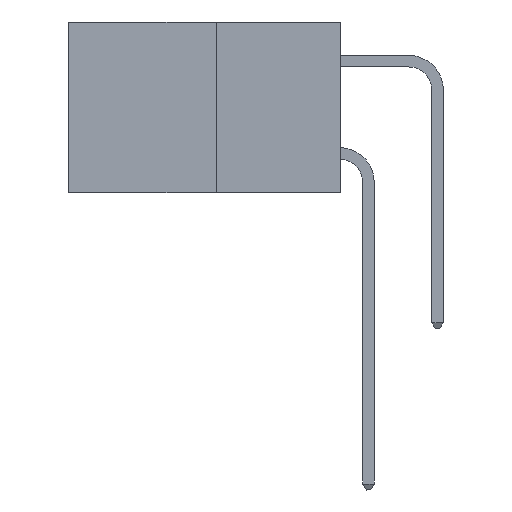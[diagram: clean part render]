
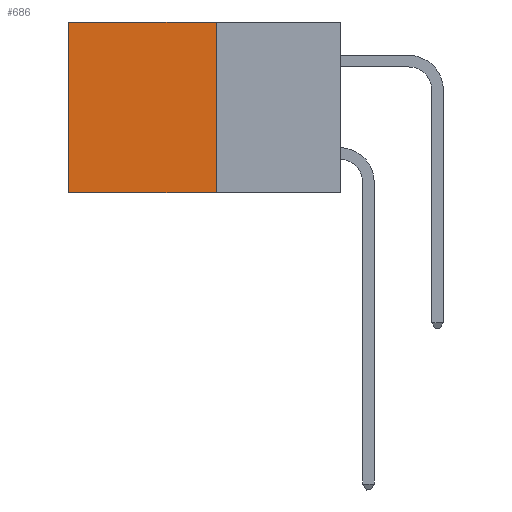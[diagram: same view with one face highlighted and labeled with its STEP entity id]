
A CAD part, left-side view. The second image highlights one B-rep face of the part: STEP entity #686.
In plain terms, the highlighted planar face has unit normal (-1, 0, 0).
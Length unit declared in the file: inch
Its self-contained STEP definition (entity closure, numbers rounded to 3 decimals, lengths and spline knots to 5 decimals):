
#374 = LINE ( 'NONE', #19249, #15645 ) ;
#686 = ADVANCED_FACE ( 'NONE', ( #7933 ), #1403, .F. ) ;
#920 = ORIENTED_EDGE ( 'NONE', *, *, #1184, .F. ) ;
#1184 = EDGE_CURVE ( 'NONE', #19077, #5666, #11790, .T. ) ;
#1374 = DIRECTION ( 'NONE',  ( 1., 0., 0. ) ) ;
#1403 = PLANE ( 'NONE',  #2639 ) ;
#1938 = CARTESIAN_POINT ( 'NONE',  ( 0.277, 0.27, -0.37 ) ) ;
#2235 = EDGE_CURVE ( 'NONE', #8948, #19077, #8151, .T. ) ;
#2639 = AXIS2_PLACEMENT_3D ( 'NONE', #1938, #1374, #23322 ) ;
#3296 = CARTESIAN_POINT ( 'NONE',  ( 0.277, 0.27, -0.37 ) ) ;
#3672 = CARTESIAN_POINT ( 'NONE',  ( 0.277, 0.59, -0.37 ) ) ;
#4010 = DIRECTION ( 'NONE',  ( 0., 0., -1. ) ) ;
#5666 = VERTEX_POINT ( 'NONE', #15657 ) ;
#6806 = DIRECTION ( 'NONE',  ( 0., 1., 0. ) ) ;
#7250 = EDGE_CURVE ( 'NONE', #21958, #5666, #17020, .T. ) ;
#7867 = DIRECTION ( 'NONE',  ( 0., 1., 0. ) ) ;
#7933 = FACE_OUTER_BOUND ( 'NONE', #14945, .T. ) ;
#8151 = LINE ( 'NONE', #12374, #17680 ) ;
#8948 = VERTEX_POINT ( 'NONE', #10159 ) ;
#9291 = ORIENTED_EDGE ( 'NONE', *, *, #2235, .F. ) ;
#9844 = CARTESIAN_POINT ( 'NONE',  ( 0.277, 0.59, 0. ) ) ;
#10159 = CARTESIAN_POINT ( 'NONE',  ( 0.277, 0.27, 0. ) ) ;
#11790 = LINE ( 'NONE', #16124, #20679 ) ;
#11961 = VECTOR ( 'NONE', #4010, 39.37008 ) ;
#12374 = CARTESIAN_POINT ( 'NONE',  ( 0.277, 0.27, -0.37 ) ) ;
#13967 = ORIENTED_EDGE ( 'NONE', *, *, #14857, .T. ) ;
#14857 = EDGE_CURVE ( 'NONE', #8948, #21958, #374, .T. ) ;
#14945 = EDGE_LOOP ( 'NONE', ( #14998, #920, #9291, #13967 ) ) ;
#14998 = ORIENTED_EDGE ( 'NONE', *, *, #7250, .T. ) ;
#15645 = VECTOR ( 'NONE', #7867, 39.37008 ) ;
#15657 = CARTESIAN_POINT ( 'NONE',  ( 0.277, 0.59, -0.37 ) ) ;
#16124 = CARTESIAN_POINT ( 'NONE',  ( 0.277, 0.27, -0.37 ) ) ;
#17020 = LINE ( 'NONE', #3672, #11961 ) ;
#17248 = DIRECTION ( 'NONE',  ( 0., 0., -1. ) ) ;
#17680 = VECTOR ( 'NONE', #17248, 39.37008 ) ;
#19077 = VERTEX_POINT ( 'NONE', #3296 ) ;
#19249 = CARTESIAN_POINT ( 'NONE',  ( 0.277, 0.27, 0. ) ) ;
#20679 = VECTOR ( 'NONE', #6806, 39.37008 ) ;
#21958 = VERTEX_POINT ( 'NONE', #9844 ) ;
#23322 = DIRECTION ( 'NONE',  ( 0., 0., -1. ) ) ;
